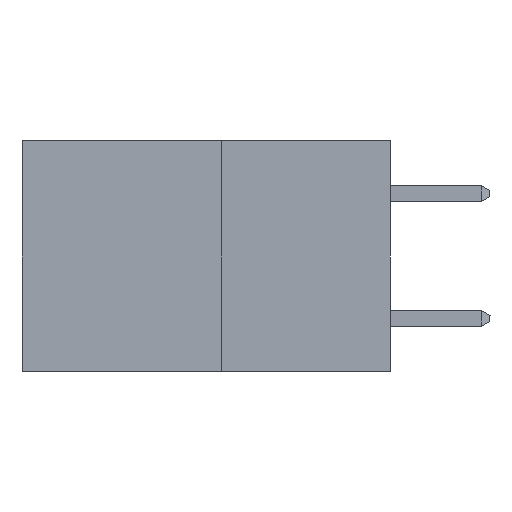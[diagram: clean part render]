
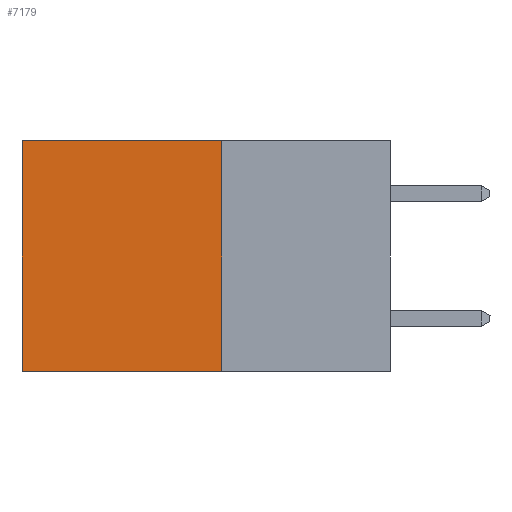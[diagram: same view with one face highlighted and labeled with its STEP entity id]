
A CAD part, left-side view. The second image highlights one B-rep face of the part: STEP entity #7179.
In plain terms, the highlighted planar face has unit normal (-1, 0, 0).
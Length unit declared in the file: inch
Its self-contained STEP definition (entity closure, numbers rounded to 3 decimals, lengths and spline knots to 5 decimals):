
#1021 = DIRECTION ( 'NONE',  ( 0., 1., 0. ) ) ;
#1075 = CARTESIAN_POINT ( 'NONE',  ( 0.277, 0.27, -0.37 ) ) ;
#1197 = VECTOR ( 'NONE', #19234, 39.37008 ) ;
#2141 = VECTOR ( 'NONE', #1021, 39.37008 ) ;
#2723 = ORIENTED_EDGE ( 'NONE', *, *, #12907, .T. ) ;
#2743 = LINE ( 'NONE', #1075, #2141 ) ;
#3365 = VERTEX_POINT ( 'NONE', #17367 ) ;
#4296 = DIRECTION ( 'NONE',  ( 0., 0., -1. ) ) ;
#4317 = CARTESIAN_POINT ( 'NONE',  ( 0.277, 0.27, 0. ) ) ;
#4328 = DIRECTION ( 'NONE',  ( 1., 0., 0. ) ) ;
#4355 = PLANE ( 'NONE',  #20005 ) ;
#4396 = CARTESIAN_POINT ( 'NONE',  ( 0.277, 0.59, -0.37 ) ) ;
#4641 = CARTESIAN_POINT ( 'NONE',  ( 0.277, 0.27, -0.37 ) ) ;
#4749 = VERTEX_POINT ( 'NONE', #12731 ) ;
#5902 = EDGE_LOOP ( 'NONE', ( #2723, #19875, #8579, #18476 ) ) ;
#6339 = EDGE_CURVE ( 'NONE', #8799, #3365, #2743, .T. ) ;
#7179 = ADVANCED_FACE ( 'NONE', ( #22975 ), #4355, .F. ) ;
#8182 = VECTOR ( 'NONE', #15344, 39.37008 ) ;
#8579 = ORIENTED_EDGE ( 'NONE', *, *, #16388, .F. ) ;
#8799 = VERTEX_POINT ( 'NONE', #17711 ) ;
#11618 = CARTESIAN_POINT ( 'NONE',  ( 0.277, 0.27, -0.37 ) ) ;
#11711 = VECTOR ( 'NONE', #22841, 39.37008 ) ;
#12302 = LINE ( 'NONE', #4317, #11711 ) ;
#12731 = CARTESIAN_POINT ( 'NONE',  ( 0.277, 0.27, 0. ) ) ;
#12907 = EDGE_CURVE ( 'NONE', #17786, #3365, #16034, .T. ) ;
#15344 = DIRECTION ( 'NONE',  ( 0., 0., -1. ) ) ;
#15695 = EDGE_CURVE ( 'NONE', #4749, #17786, #12302, .T. ) ;
#16034 = LINE ( 'NONE', #4396, #1197 ) ;
#16388 = EDGE_CURVE ( 'NONE', #4749, #8799, #22918, .T. ) ;
#17367 = CARTESIAN_POINT ( 'NONE',  ( 0.277, 0.59, -0.37 ) ) ;
#17711 = CARTESIAN_POINT ( 'NONE',  ( 0.277, 0.27, -0.37 ) ) ;
#17786 = VERTEX_POINT ( 'NONE', #18589 ) ;
#18476 = ORIENTED_EDGE ( 'NONE', *, *, #15695, .T. ) ;
#18589 = CARTESIAN_POINT ( 'NONE',  ( 0.277, 0.59, 0. ) ) ;
#19234 = DIRECTION ( 'NONE',  ( 0., 0., -1. ) ) ;
#19875 = ORIENTED_EDGE ( 'NONE', *, *, #6339, .F. ) ;
#20005 = AXIS2_PLACEMENT_3D ( 'NONE', #4641, #4328, #4296 ) ;
#22841 = DIRECTION ( 'NONE',  ( 0., 1., 0. ) ) ;
#22918 = LINE ( 'NONE', #11618, #8182 ) ;
#22975 = FACE_OUTER_BOUND ( 'NONE', #5902, .T. ) ;
